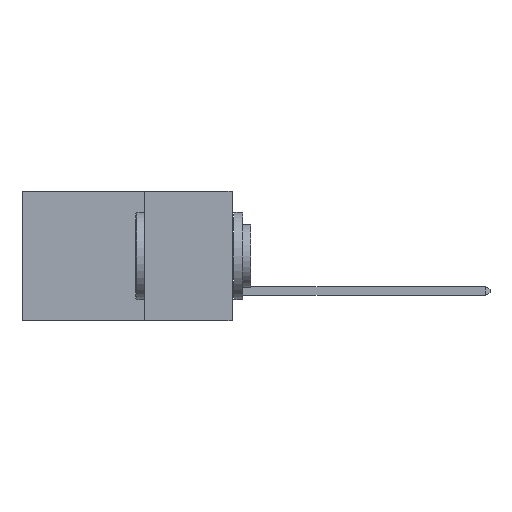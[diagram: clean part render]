
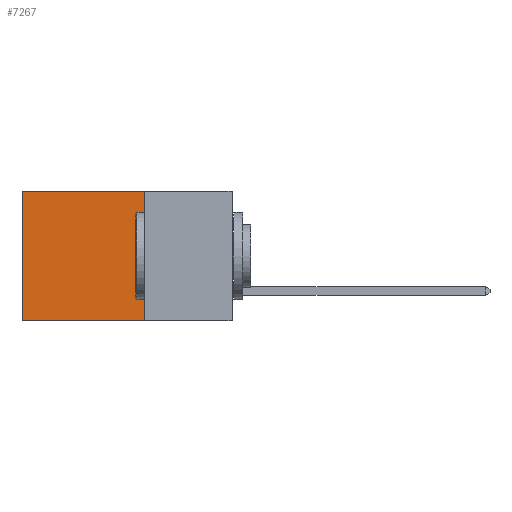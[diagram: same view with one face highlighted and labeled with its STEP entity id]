
A CAD part, left-side view. The second image highlights one B-rep face of the part: STEP entity #7267.
In plain terms, the highlighted planar face has unit normal (-1, 0, 0).
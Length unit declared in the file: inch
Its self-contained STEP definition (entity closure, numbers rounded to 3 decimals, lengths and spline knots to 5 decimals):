
#46 = VECTOR ( 'NONE', #11877, 39.37008 ) ;
#2352 = EDGE_CURVE ( 'NONE', #39738, #39113, #32441, .T. ) ;
#3419 = LINE ( 'NONE', #37139, #32924 ) ;
#3492 = DIRECTION ( 'NONE',  ( 0., 0., -1. ) ) ;
#4065 = DIRECTION ( 'NONE',  ( 1., 0., 0. ) ) ;
#4323 = DIRECTION ( 'NONE',  ( 0., 0., -1. ) ) ;
#5161 = LINE ( 'NONE', #5209, #46 ) ;
#5209 = CARTESIAN_POINT ( 'NONE',  ( 0.2875, 0.25, 0. ) ) ;
#5743 = CARTESIAN_POINT ( 'NONE',  ( 0.2875, 0.6, 0. ) ) ;
#6023 = LINE ( 'NONE', #34867, #14678 ) ;
#7267 = ADVANCED_FACE ( 'NONE', ( #39466 ), #33236, .F. ) ;
#7871 = AXIS2_PLACEMENT_3D ( 'NONE', #23564, #4065, #4323 ) ;
#10322 = EDGE_CURVE ( 'NONE', #11712, #23150, #6023, .T. ) ;
#11712 = VERTEX_POINT ( 'NONE', #5743 ) ;
#11877 = DIRECTION ( 'NONE',  ( 0., 1., 0. ) ) ;
#14678 = VECTOR ( 'NONE', #25050, 39.37008 ) ;
#16202 = ORIENTED_EDGE ( 'NONE', *, *, #16420, .T. ) ;
#16420 = EDGE_CURVE ( 'NONE', #39738, #11712, #5161, .T. ) ;
#16927 = CARTESIAN_POINT ( 'NONE',  ( 0.2875, 0.25, -0.37 ) ) ;
#18111 = ORIENTED_EDGE ( 'NONE', *, *, #18735, .F. ) ;
#18735 = EDGE_CURVE ( 'NONE', #39113, #23150, #3419, .T. ) ;
#22903 = ORIENTED_EDGE ( 'NONE', *, *, #10322, .T. ) ;
#22992 = CARTESIAN_POINT ( 'NONE',  ( 0.2875, 0.25, 0. ) ) ;
#23150 = VERTEX_POINT ( 'NONE', #27863 ) ;
#23564 = CARTESIAN_POINT ( 'NONE',  ( 0.2875, 0.25, 0. ) ) ;
#24219 = DIRECTION ( 'NONE',  ( 0., 1., 0. ) ) ;
#25050 = DIRECTION ( 'NONE',  ( 0., 0., -1. ) ) ;
#27848 = EDGE_LOOP ( 'NONE', ( #22903, #18111, #38578, #16202 ) ) ;
#27863 = CARTESIAN_POINT ( 'NONE',  ( 0.2875, 0.6, -0.37 ) ) ;
#32441 = LINE ( 'NONE', #22992, #39491 ) ;
#32924 = VECTOR ( 'NONE', #24219, 39.37008 ) ;
#33236 = PLANE ( 'NONE',  #7871 ) ;
#34867 = CARTESIAN_POINT ( 'NONE',  ( 0.2875, 0.6, 0. ) ) ;
#37139 = CARTESIAN_POINT ( 'NONE',  ( 0.2875, 0.25, -0.37 ) ) ;
#38578 = ORIENTED_EDGE ( 'NONE', *, *, #2352, .F. ) ;
#39113 = VERTEX_POINT ( 'NONE', #16927 ) ;
#39466 = FACE_OUTER_BOUND ( 'NONE', #27848, .T. ) ;
#39491 = VECTOR ( 'NONE', #3492, 39.37008 ) ;
#39738 = VERTEX_POINT ( 'NONE', #41507 ) ;
#41507 = CARTESIAN_POINT ( 'NONE',  ( 0.2875, 0.25, 0. ) ) ;
